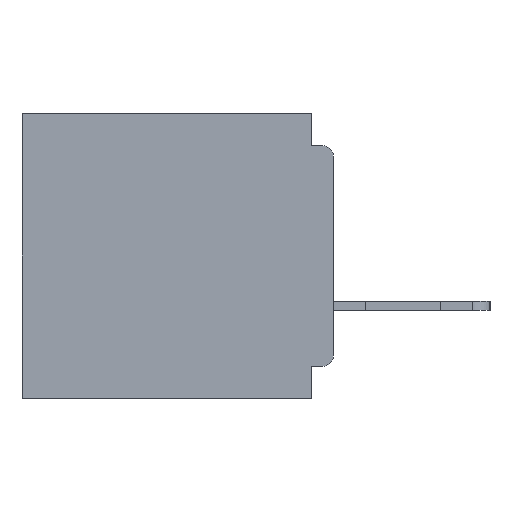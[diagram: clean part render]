
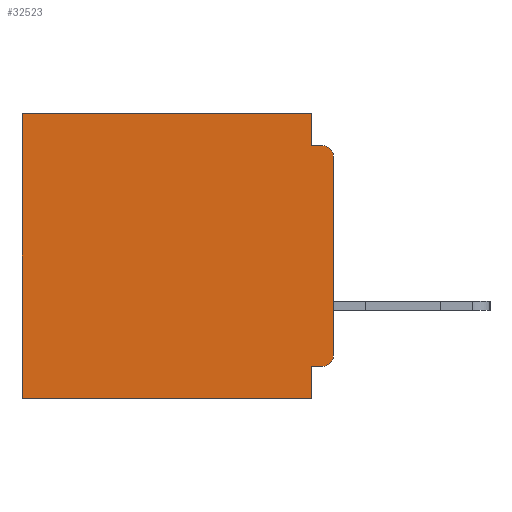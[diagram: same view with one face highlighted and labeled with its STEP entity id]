
A CAD part, left-side view. The second image highlights one B-rep face of the part: STEP entity #32523.
In plain terms, the highlighted planar face has unit normal (-1, 0, 0).
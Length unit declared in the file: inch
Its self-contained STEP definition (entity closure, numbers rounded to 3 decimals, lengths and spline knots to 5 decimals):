
#748 = VERTEX_POINT ( 'NONE', #45095 ) ;
#1271 = VERTEX_POINT ( 'NONE', #18200 ) ;
#1410 = EDGE_CURVE ( 'NONE', #748, #1271, #37829, .T. ) ;
#1725 = PLANE ( 'NONE',  #14275 ) ;
#2012 = CARTESIAN_POINT ( 'NONE',  ( 0.3, 0.437, -0.4 ) ) ;
#2266 = CARTESIAN_POINT ( 'NONE',  ( 0.3, 0., -0.355 ) ) ;
#3235 = AXIS2_PLACEMENT_3D ( 'NONE', #53759, #53620, #53636 ) ;
#3538 = EDGE_CURVE ( 'NONE', #748, #23675, #48879, .T. ) ;
#3556 = EDGE_CURVE ( 'NONE', #11563, #45608, #14971, .T. ) ;
#4447 = VECTOR ( 'NONE', #55788, 39.37008 ) ;
#4498 = DIRECTION ( 'NONE',  ( 0., 0., -1. ) ) ;
#4561 = EDGE_CURVE ( 'NONE', #11563, #22123, #54960, .T. ) ;
#7945 = EDGE_CURVE ( 'NONE', #23675, #56856, #15101, .T. ) ;
#9094 = ORIENTED_EDGE ( 'NONE', *, *, #34831, .F. ) ;
#9182 = DIRECTION ( 'NONE',  ( -1., 0., 0. ) ) ;
#11269 = EDGE_CURVE ( 'NONE', #51856, #41180, #43548, .T. ) ;
#11563 = VERTEX_POINT ( 'NONE', #55265 ) ;
#14275 = AXIS2_PLACEMENT_3D ( 'NONE', #54887, #41649, #32954 ) ;
#14339 = VERTEX_POINT ( 'NONE', #56379 ) ;
#14971 = CIRCLE ( 'NONE', #3235, 0.015 ) ;
#15101 = LINE ( 'NONE', #40562, #37322 ) ;
#16386 = CARTESIAN_POINT ( 'NONE',  ( 0.3, 0., -0.4 ) ) ;
#18200 = CARTESIAN_POINT ( 'NONE',  ( 0.3, 0.031, -0.045 ) ) ;
#18913 = ORIENTED_EDGE ( 'NONE', *, *, #36963, .F. ) ;
#19022 = DIRECTION ( 'NONE',  ( 0., 0., -1. ) ) ;
#19743 = FACE_OUTER_BOUND ( 'NONE', #52176, .T. ) ;
#21096 = ORIENTED_EDGE ( 'NONE', *, *, #3538, .T. ) ;
#21961 = LINE ( 'NONE', #45550, #45497 ) ;
#22123 = VERTEX_POINT ( 'NONE', #26827 ) ;
#22425 = VECTOR ( 'NONE', #29781, 39.37008 ) ;
#22610 = CARTESIAN_POINT ( 'NONE',  ( 0.3, 0., -0.045 ) ) ;
#23337 = ORIENTED_EDGE ( 'NONE', *, *, #3556, .T. ) ;
#23675 = VERTEX_POINT ( 'NONE', #25581 ) ;
#23815 = AXIS2_PLACEMENT_3D ( 'NONE', #35861, #9182, #40311 ) ;
#25581 = CARTESIAN_POINT ( 'NONE',  ( 0.3, 0.437, 0. ) ) ;
#26827 = CARTESIAN_POINT ( 'NONE',  ( 0.3, 0.031, -0.355 ) ) ;
#27090 = DIRECTION ( 'NONE',  ( 0., -1., 0. ) ) ;
#27484 = VECTOR ( 'NONE', #4498, 39.37008 ) ;
#28242 = LINE ( 'NONE', #51324, #4447 ) ;
#28786 = ORIENTED_EDGE ( 'NONE', *, *, #11269, .T. ) ;
#29321 = VECTOR ( 'NONE', #27090, 39.37008 ) ;
#29781 = DIRECTION ( 'NONE',  ( 0., 1., 0. ) ) ;
#31502 = EDGE_CURVE ( 'NONE', #51856, #45608, #28242, .T. ) ;
#32523 = ADVANCED_FACE ( 'NONE', ( #19743 ), #1725, .F. ) ;
#32791 = ORIENTED_EDGE ( 'NONE', *, *, #7945, .T. ) ;
#32954 = DIRECTION ( 'NONE',  ( 0., 0., -1. ) ) ;
#34831 = EDGE_CURVE ( 'NONE', #22123, #14339, #21961, .T. ) ;
#35820 = VECTOR ( 'NONE', #55735, 39.37008 ) ;
#35861 = CARTESIAN_POINT ( 'NONE',  ( 0.3, 0.015, -0.06 ) ) ;
#36126 = DIRECTION ( 'NONE',  ( 0., 0., -1. ) ) ;
#36614 = ORIENTED_EDGE ( 'NONE', *, *, #4561, .F. ) ;
#36963 = EDGE_CURVE ( 'NONE', #1271, #41180, #41084, .T. ) ;
#37322 = VECTOR ( 'NONE', #36126, 39.37008 ) ;
#37829 = LINE ( 'NONE', #56118, #27484 ) ;
#40311 = DIRECTION ( 'NONE',  ( 0., 0., -1. ) ) ;
#40562 = CARTESIAN_POINT ( 'NONE',  ( 0.3, 0.437, -0.4 ) ) ;
#40692 = CARTESIAN_POINT ( 'NONE',  ( 0.3, 0., -0.34 ) ) ;
#41084 = LINE ( 'NONE', #22610, #29321 ) ;
#41180 = VERTEX_POINT ( 'NONE', #47009 ) ;
#41649 = DIRECTION ( 'NONE',  ( 1., 0., 0. ) ) ;
#43548 = CIRCLE ( 'NONE', #23815, 0.015 ) ;
#45095 = CARTESIAN_POINT ( 'NONE',  ( 0.3, 0.031, 0. ) ) ;
#45497 = VECTOR ( 'NONE', #19022, 39.37008 ) ;
#45550 = CARTESIAN_POINT ( 'NONE',  ( 0.3, 0.031, -0.4 ) ) ;
#45608 = VERTEX_POINT ( 'NONE', #40692 ) ;
#45943 = LINE ( 'NONE', #16386, #22425 ) ;
#47009 = CARTESIAN_POINT ( 'NONE',  ( 0.3, 0.015, -0.045 ) ) ;
#48764 = ORIENTED_EDGE ( 'NONE', *, *, #1410, .F. ) ;
#48879 = LINE ( 'NONE', #57154, #35820 ) ;
#50100 = ORIENTED_EDGE ( 'NONE', *, *, #51355, .F. ) ;
#51273 = CARTESIAN_POINT ( 'NONE',  ( 0.3, 0., -0.06 ) ) ;
#51324 = CARTESIAN_POINT ( 'NONE',  ( 0.3, 0., -0.4 ) ) ;
#51355 = EDGE_CURVE ( 'NONE', #14339, #56856, #45943, .T. ) ;
#51856 = VERTEX_POINT ( 'NONE', #51273 ) ;
#52176 = EDGE_LOOP ( 'NONE', ( #55753, #28786, #18913, #48764, #21096, #32791, #50100, #9094, #36614, #23337 ) ) ;
#52183 = VECTOR ( 'NONE', #56472, 39.37008 ) ;
#53620 = DIRECTION ( 'NONE',  ( -1., 0., 0. ) ) ;
#53636 = DIRECTION ( 'NONE',  ( 0., 0., -1. ) ) ;
#53759 = CARTESIAN_POINT ( 'NONE',  ( 0.3, 0.015, -0.34 ) ) ;
#54887 = CARTESIAN_POINT ( 'NONE',  ( 0.3, 0., -0.4 ) ) ;
#54960 = LINE ( 'NONE', #2266, #52183 ) ;
#55265 = CARTESIAN_POINT ( 'NONE',  ( 0.3, 0.015, -0.355 ) ) ;
#55735 = DIRECTION ( 'NONE',  ( 0., 1., 0. ) ) ;
#55753 = ORIENTED_EDGE ( 'NONE', *, *, #31502, .F. ) ;
#55788 = DIRECTION ( 'NONE',  ( 0., 0., -1. ) ) ;
#56118 = CARTESIAN_POINT ( 'NONE',  ( 0.3, 0.031, 0. ) ) ;
#56379 = CARTESIAN_POINT ( 'NONE',  ( 0.3, 0.031, -0.4 ) ) ;
#56472 = DIRECTION ( 'NONE',  ( 0., 1., 0. ) ) ;
#56856 = VERTEX_POINT ( 'NONE', #2012 ) ;
#57154 = CARTESIAN_POINT ( 'NONE',  ( 0.3, 0., 0. ) ) ;
